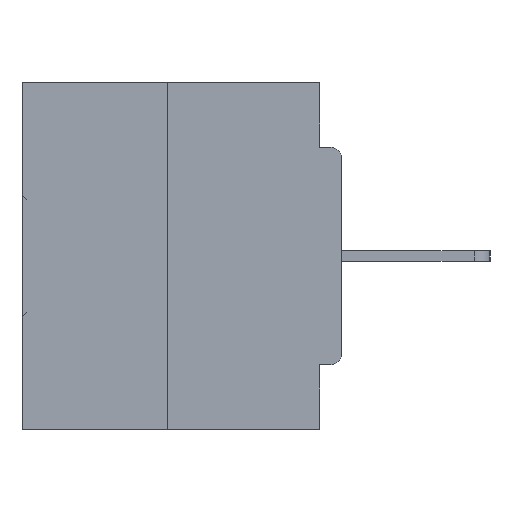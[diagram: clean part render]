
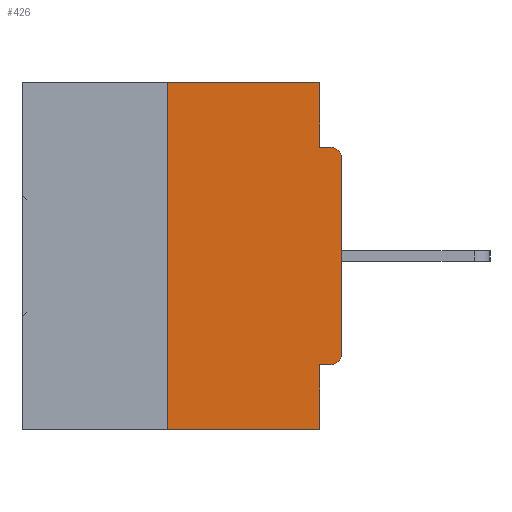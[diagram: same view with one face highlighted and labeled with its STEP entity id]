
A CAD part, left-side view. The second image highlights one B-rep face of the part: STEP entity #426.
In plain terms, the highlighted planar face has unit normal (-1, 0, 0).
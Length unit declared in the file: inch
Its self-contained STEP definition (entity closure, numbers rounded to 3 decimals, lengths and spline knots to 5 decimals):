
#261 = CARTESIAN_POINT ( 'NONE',  ( 0., 0.031, -0.5 ) ) ;
#421 = EDGE_CURVE ( 'NONE', #13317, #24622, #16438, .T. ) ;
#426 = ADVANCED_FACE ( 'NONE', ( #4825 ), #25837, .F. ) ;
#433 = EDGE_CURVE ( 'NONE', #27221, #35513, #7857, .T. ) ;
#718 = VECTOR ( 'NONE', #21380, 39.37008 ) ;
#1184 = DIRECTION ( 'NONE',  ( 0., 0., -1. ) ) ;
#1673 = EDGE_CURVE ( 'NONE', #35513, #24622, #5623, .T. ) ;
#2435 = DIRECTION ( 'NONE',  ( -1., 0., 0. ) ) ;
#2645 = CARTESIAN_POINT ( 'NONE',  ( 0., 0., -0.4065 ) ) ;
#3029 = VECTOR ( 'NONE', #5916, 39.37008 ) ;
#3756 = ORIENTED_EDGE ( 'NONE', *, *, #433, .T. ) ;
#3992 = EDGE_CURVE ( 'NONE', #19957, #26607, #30485, .T. ) ;
#4226 = DIRECTION ( 'NONE',  ( 0., -1., 0. ) ) ;
#4289 = CARTESIAN_POINT ( 'NONE',  ( 0., 0.015, -0.0935 ) ) ;
#4825 = FACE_OUTER_BOUND ( 'NONE', #16450, .T. ) ;
#5623 = CIRCLE ( 'NONE', #9477, 0.015 ) ;
#5900 = VECTOR ( 'NONE', #4226, 39.37008 ) ;
#5916 = DIRECTION ( 'NONE',  ( 0., -1., 0. ) ) ;
#6229 = VERTEX_POINT ( 'NONE', #25188 ) ;
#6305 = DIRECTION ( 'NONE',  ( 0., 0., 1. ) ) ;
#6516 = ORIENTED_EDGE ( 'NONE', *, *, #26327, .F. ) ;
#6547 = ORIENTED_EDGE ( 'NONE', *, *, #18348, .F. ) ;
#6637 = CARTESIAN_POINT ( 'NONE',  ( 0., 0.25, 0. ) ) ;
#6648 = DIRECTION ( 'NONE',  ( 0., 0., -1. ) ) ;
#7340 = CARTESIAN_POINT ( 'NONE',  ( 0., 0.031, 0. ) ) ;
#7449 = EDGE_CURVE ( 'NONE', #6229, #36243, #33850, .T. ) ;
#7857 = LINE ( 'NONE', #13059, #21234 ) ;
#8125 = EDGE_CURVE ( 'NONE', #19957, #36243, #35714, .T. ) ;
#9477 = AXIS2_PLACEMENT_3D ( 'NONE', #23437, #2435, #38843 ) ;
#10866 = CARTESIAN_POINT ( 'NONE',  ( 0., 0.031, 0. ) ) ;
#11326 = VECTOR ( 'NONE', #6648, 39.37008 ) ;
#11576 = CARTESIAN_POINT ( 'NONE',  ( 0., 0.015, -0.4065 ) ) ;
#11855 = CARTESIAN_POINT ( 'NONE',  ( 0., 0.031, -0.5 ) ) ;
#12502 = AXIS2_PLACEMENT_3D ( 'NONE', #31572, #28360, #1184 ) ;
#12674 = ORIENTED_EDGE ( 'NONE', *, *, #421, .F. ) ;
#13059 = CARTESIAN_POINT ( 'NONE',  ( 0., 0., 0. ) ) ;
#13317 = VERTEX_POINT ( 'NONE', #34882 ) ;
#14785 = CARTESIAN_POINT ( 'NONE',  ( 0., 0.46, 0. ) ) ;
#14871 = ORIENTED_EDGE ( 'NONE', *, *, #7449, .F. ) ;
#15302 = CARTESIAN_POINT ( 'NONE',  ( 0., 0.25, 0. ) ) ;
#16247 = DIRECTION ( 'NONE',  ( 0., 0., 1. ) ) ;
#16438 = LINE ( 'NONE', #32239, #5900 ) ;
#16450 = EDGE_LOOP ( 'NONE', ( #24959, #38186, #21152, #14871, #6547, #24113, #3756, #25607, #12674, #6516 ) ) ;
#16645 = DIRECTION ( 'NONE',  ( 1., 0., 0. ) ) ;
#17030 = CARTESIAN_POINT ( 'NONE',  ( 0., 0.46, 0. ) ) ;
#17216 = VECTOR ( 'NONE', #32261, 39.37008 ) ;
#18230 = CIRCLE ( 'NONE', #12502, 0.015 ) ;
#18348 = EDGE_CURVE ( 'NONE', #36998, #6229, #30035, .T. ) ;
#19957 = VERTEX_POINT ( 'NONE', #22495 ) ;
#20745 = VECTOR ( 'NONE', #6305, 39.37008 ) ;
#21113 = CARTESIAN_POINT ( 'NONE',  ( 0., 0.46, -0.5 ) ) ;
#21152 = ORIENTED_EDGE ( 'NONE', *, *, #8125, .T. ) ;
#21234 = VECTOR ( 'NONE', #16247, 39.37008 ) ;
#21380 = DIRECTION ( 'NONE',  ( 0., -1., 0. ) ) ;
#22495 = CARTESIAN_POINT ( 'NONE',  ( 0., 0.25, -0.5 ) ) ;
#23437 = CARTESIAN_POINT ( 'NONE',  ( 0., 0.015, -0.1085 ) ) ;
#23864 = EDGE_CURVE ( 'NONE', #26607, #37202, #23975, .T. ) ;
#23975 = LINE ( 'NONE', #14785, #718 ) ;
#24113 = ORIENTED_EDGE ( 'NONE', *, *, #37941, .T. ) ;
#24622 = VERTEX_POINT ( 'NONE', #4289 ) ;
#24959 = ORIENTED_EDGE ( 'NONE', *, *, #23864, .F. ) ;
#25188 = CARTESIAN_POINT ( 'NONE',  ( 0., 0.031, -0.4065 ) ) ;
#25607 = ORIENTED_EDGE ( 'NONE', *, *, #1673, .T. ) ;
#25837 = PLANE ( 'NONE',  #28232 ) ;
#26327 = EDGE_CURVE ( 'NONE', #37202, #13317, #38251, .T. ) ;
#26607 = VERTEX_POINT ( 'NONE', #6637 ) ;
#27221 = VERTEX_POINT ( 'NONE', #37251 ) ;
#28115 = CARTESIAN_POINT ( 'NONE',  ( 0., 0., -0.1085 ) ) ;
#28232 = AXIS2_PLACEMENT_3D ( 'NONE', #17030, #16645, #35234 ) ;
#28360 = DIRECTION ( 'NONE',  ( -1., 0., 0. ) ) ;
#30035 = LINE ( 'NONE', #2645, #30672 ) ;
#30485 = LINE ( 'NONE', #15302, #20745 ) ;
#30672 = VECTOR ( 'NONE', #32850, 39.37008 ) ;
#31572 = CARTESIAN_POINT ( 'NONE',  ( 0., 0.015, -0.3915 ) ) ;
#32239 = CARTESIAN_POINT ( 'NONE',  ( 0., 0., -0.0935 ) ) ;
#32261 = DIRECTION ( 'NONE',  ( 0., 0., -1. ) ) ;
#32850 = DIRECTION ( 'NONE',  ( 0., 1., 0. ) ) ;
#33850 = LINE ( 'NONE', #261, #11326 ) ;
#34882 = CARTESIAN_POINT ( 'NONE',  ( 0., 0.031, -0.0935 ) ) ;
#35234 = DIRECTION ( 'NONE',  ( 0., 0., -1. ) ) ;
#35513 = VERTEX_POINT ( 'NONE', #28115 ) ;
#35714 = LINE ( 'NONE', #21113, #3029 ) ;
#36243 = VERTEX_POINT ( 'NONE', #11855 ) ;
#36998 = VERTEX_POINT ( 'NONE', #11576 ) ;
#37202 = VERTEX_POINT ( 'NONE', #7340 ) ;
#37251 = CARTESIAN_POINT ( 'NONE',  ( 0., 0., -0.3915 ) ) ;
#37941 = EDGE_CURVE ( 'NONE', #36998, #27221, #18230, .T. ) ;
#38186 = ORIENTED_EDGE ( 'NONE', *, *, #3992, .F. ) ;
#38251 = LINE ( 'NONE', #10866, #17216 ) ;
#38843 = DIRECTION ( 'NONE',  ( 0., 0., -1. ) ) ;
